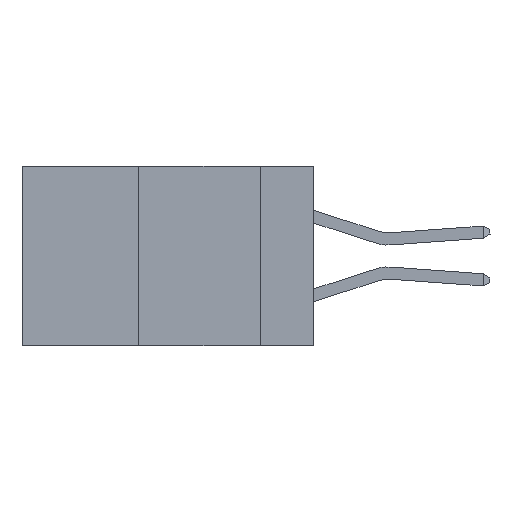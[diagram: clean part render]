
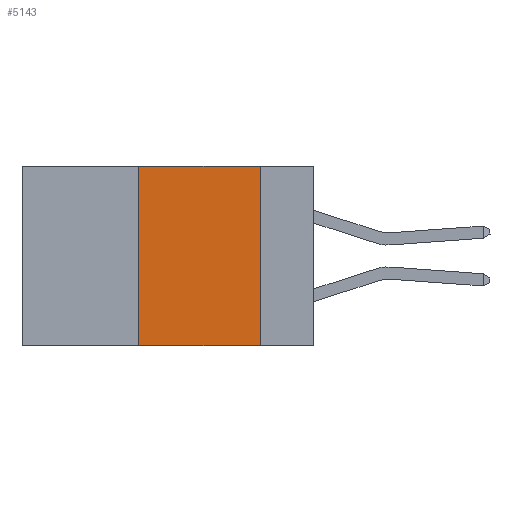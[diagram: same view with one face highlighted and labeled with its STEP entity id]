
A CAD part, left-side view. The second image highlights one B-rep face of the part: STEP entity #5143.
In plain terms, the highlighted planar face has unit normal (-1, 0, 0).
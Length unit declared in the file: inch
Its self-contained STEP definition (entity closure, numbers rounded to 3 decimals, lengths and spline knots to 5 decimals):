
#65 = ORIENTED_EDGE ( 'NONE', *, *, #4628, .F. ) ;
#459 = CARTESIAN_POINT ( 'NONE',  ( 0., 0.36, 0. ) ) ;
#607 = VERTEX_POINT ( 'NONE', #459 ) ;
#1247 = CARTESIAN_POINT ( 'NONE',  ( 0., 0.6, 0. ) ) ;
#1268 = ORIENTED_EDGE ( 'NONE', *, *, #6441, .F. ) ;
#1313 = VERTEX_POINT ( 'NONE', #11008 ) ;
#1325 = DIRECTION ( 'NONE',  ( 0., -1., 0. ) ) ;
#1356 = DIRECTION ( 'NONE',  ( 0., 0., -1. ) ) ;
#2313 = VECTOR ( 'NONE', #1325, 39.37008 ) ;
#3317 = CARTESIAN_POINT ( 'NONE',  ( 0., 0.6, -0.37 ) ) ;
#4600 = VECTOR ( 'NONE', #10064, 39.37008 ) ;
#4628 = EDGE_CURVE ( 'NONE', #7489, #607, #7785, .T. ) ;
#4727 = DIRECTION ( 'NONE',  ( 1., 0., 0. ) ) ;
#5143 = ADVANCED_FACE ( 'NONE', ( #9244 ), #11578, .F. ) ;
#5597 = CARTESIAN_POINT ( 'NONE',  ( 0., 0.36, 0. ) ) ;
#6019 = EDGE_LOOP ( 'NONE', ( #1268, #6550, #65, #8073 ) ) ;
#6441 = EDGE_CURVE ( 'NONE', #1313, #6850, #10626, .T. ) ;
#6550 = ORIENTED_EDGE ( 'NONE', *, *, #13501, .F. ) ;
#6850 = VERTEX_POINT ( 'NONE', #14114 ) ;
#7489 = VERTEX_POINT ( 'NONE', #7594 ) ;
#7594 = CARTESIAN_POINT ( 'NONE',  ( 0., 0.36, -0.37 ) ) ;
#7785 = LINE ( 'NONE', #5597, #4600 ) ;
#8073 = ORIENTED_EDGE ( 'NONE', *, *, #11122, .T. ) ;
#8274 = CARTESIAN_POINT ( 'NONE',  ( 0., 0.11, 0. ) ) ;
#9136 = VECTOR ( 'NONE', #9312, 39.37008 ) ;
#9244 = FACE_OUTER_BOUND ( 'NONE', #6019, .T. ) ;
#9312 = DIRECTION ( 'NONE',  ( 0., -1., 0. ) ) ;
#10064 = DIRECTION ( 'NONE',  ( 0., 0., 1. ) ) ;
#10626 = LINE ( 'NONE', #8274, #13674 ) ;
#11008 = CARTESIAN_POINT ( 'NONE',  ( 0., 0.11, 0. ) ) ;
#11122 = EDGE_CURVE ( 'NONE', #7489, #6850, #11798, .T. ) ;
#11578 = PLANE ( 'NONE',  #13921 ) ;
#11798 = LINE ( 'NONE', #3317, #9136 ) ;
#13501 = EDGE_CURVE ( 'NONE', #607, #1313, #14498, .T. ) ;
#13674 = VECTOR ( 'NONE', #1356, 39.37008 ) ;
#13921 = AXIS2_PLACEMENT_3D ( 'NONE', #14006, #4727, #15329 ) ;
#14006 = CARTESIAN_POINT ( 'NONE',  ( 0., 0.6, 0. ) ) ;
#14114 = CARTESIAN_POINT ( 'NONE',  ( 0., 0.11, -0.37 ) ) ;
#14498 = LINE ( 'NONE', #1247, #2313 ) ;
#15329 = DIRECTION ( 'NONE',  ( 0., 0., -1. ) ) ;
